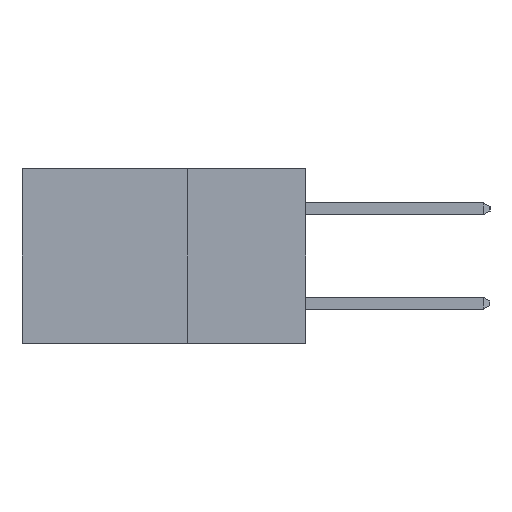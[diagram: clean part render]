
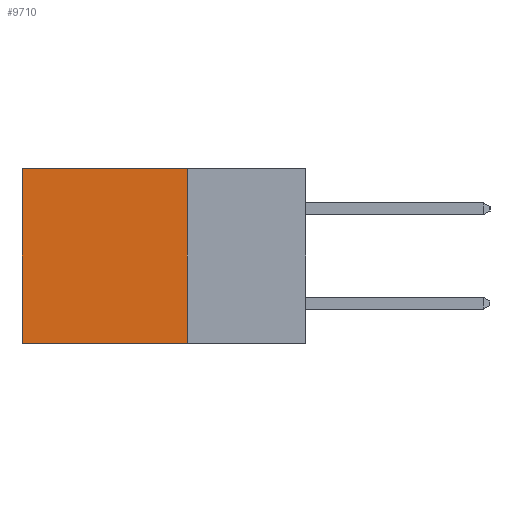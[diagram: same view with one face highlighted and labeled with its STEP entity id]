
A CAD part, left-side view. The second image highlights one B-rep face of the part: STEP entity #9710.
In plain terms, the highlighted planar face has unit normal (-1, 0, 0).
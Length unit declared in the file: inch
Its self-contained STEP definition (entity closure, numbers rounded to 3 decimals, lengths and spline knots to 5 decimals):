
#210 = DIRECTION ( 'NONE',  ( 1., 0., 0. ) ) ;
#514 = EDGE_CURVE ( 'NONE', #21201, #2978, #3580, .T. ) ;
#2801 = ORIENTED_EDGE ( 'NONE', *, *, #6403, .F. ) ;
#2978 = VERTEX_POINT ( 'NONE', #20036 ) ;
#3580 = LINE ( 'NONE', #18597, #7572 ) ;
#4381 = DIRECTION ( 'NONE',  ( 0., 0., -1. ) ) ;
#4425 = CARTESIAN_POINT ( 'NONE',  ( 0.298, 0.25, 0. ) ) ;
#4759 = CARTESIAN_POINT ( 'NONE',  ( 0.298, 0.6, -0.37 ) ) ;
#5083 = CARTESIAN_POINT ( 'NONE',  ( 0.298, 0.25, 0. ) ) ;
#5360 = VECTOR ( 'NONE', #20689, 39.37008 ) ;
#5539 = ORIENTED_EDGE ( 'NONE', *, *, #14531, .T. ) ;
#6403 = EDGE_CURVE ( 'NONE', #21201, #12748, #10987, .T. ) ;
#7233 = ORIENTED_EDGE ( 'NONE', *, *, #514, .T. ) ;
#7460 = CARTESIAN_POINT ( 'NONE',  ( 0.298, 0.25, -0.37 ) ) ;
#7572 = VECTOR ( 'NONE', #20486, 39.37008 ) ;
#9710 = ADVANCED_FACE ( 'NONE', ( #17209 ), #18590, .F. ) ;
#9904 = LINE ( 'NONE', #7460, #5360 ) ;
#10987 = LINE ( 'NONE', #4425, #14841 ) ;
#12086 = DIRECTION ( 'NONE',  ( 0., 0., -1. ) ) ;
#12243 = AXIS2_PLACEMENT_3D ( 'NONE', #13669, #210, #12086 ) ;
#12287 = VERTEX_POINT ( 'NONE', #4759 ) ;
#12748 = VERTEX_POINT ( 'NONE', #19152 ) ;
#13669 = CARTESIAN_POINT ( 'NONE',  ( 0.298, 0.25, 0. ) ) ;
#13898 = VECTOR ( 'NONE', #21390, 39.37008 ) ;
#14531 = EDGE_CURVE ( 'NONE', #2978, #12287, #18748, .T. ) ;
#14841 = VECTOR ( 'NONE', #4381, 39.37008 ) ;
#16970 = EDGE_LOOP ( 'NONE', ( #5539, #18322, #2801, #7233 ) ) ;
#17209 = FACE_OUTER_BOUND ( 'NONE', #16970, .T. ) ;
#17886 = EDGE_CURVE ( 'NONE', #12748, #12287, #9904, .T. ) ;
#18322 = ORIENTED_EDGE ( 'NONE', *, *, #17886, .F. ) ;
#18590 = PLANE ( 'NONE',  #12243 ) ;
#18597 = CARTESIAN_POINT ( 'NONE',  ( 0.298, 0.25, 0. ) ) ;
#18748 = LINE ( 'NONE', #19776, #13898 ) ;
#19152 = CARTESIAN_POINT ( 'NONE',  ( 0.298, 0.25, -0.37 ) ) ;
#19776 = CARTESIAN_POINT ( 'NONE',  ( 0.298, 0.6, 0. ) ) ;
#20036 = CARTESIAN_POINT ( 'NONE',  ( 0.298, 0.6, 0. ) ) ;
#20486 = DIRECTION ( 'NONE',  ( 0., 1., 0. ) ) ;
#20689 = DIRECTION ( 'NONE',  ( 0., 1., 0. ) ) ;
#21201 = VERTEX_POINT ( 'NONE', #5083 ) ;
#21390 = DIRECTION ( 'NONE',  ( 0., 0., -1. ) ) ;
